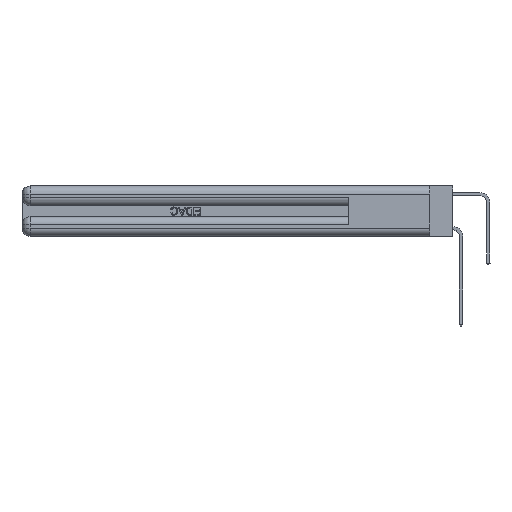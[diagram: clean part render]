
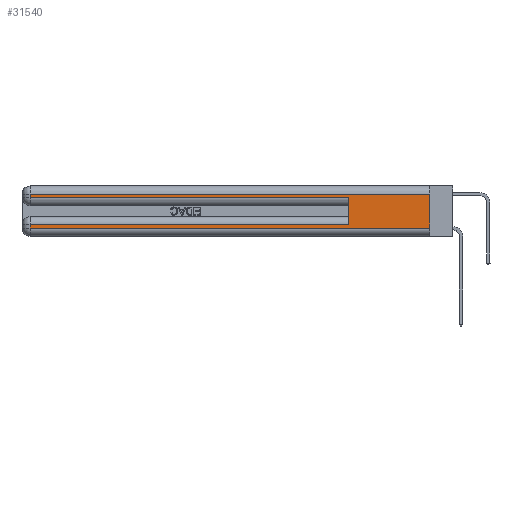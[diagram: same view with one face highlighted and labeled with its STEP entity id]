
A CAD part, left-side view. The second image highlights one B-rep face of the part: STEP entity #31540.
In plain terms, the highlighted planar face has unit normal (-1, 0, 0).
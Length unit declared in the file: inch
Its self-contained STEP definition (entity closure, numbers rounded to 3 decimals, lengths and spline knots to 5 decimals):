
#70 = CARTESIAN_POINT ( 'NONE',  ( 0., 0.6, 0.285 ) ) ;
#547 = DIRECTION ( 'NONE',  ( 0., 0., -1. ) ) ;
#630 = CARTESIAN_POINT ( 'NONE',  ( 0., 2.94, 0.06 ) ) ;
#1908 = VERTEX_POINT ( 'NONE', #31203 ) ;
#2025 = AXIS2_PLACEMENT_3D ( 'NONE', #29308, #29480, #26741 ) ;
#2280 = LINE ( 'NONE', #9863, #27321 ) ;
#4072 = ORIENTED_EDGE ( 'NONE', *, *, #21065, .T. ) ;
#4826 = LINE ( 'NONE', #23389, #30517 ) ;
#4921 = LINE ( 'NONE', #17316, #7144 ) ;
#6355 = EDGE_CURVE ( 'NONE', #16279, #23256, #4921, .T. ) ;
#6655 = EDGE_CURVE ( 'NONE', #13096, #23256, #31890, .T. ) ;
#7144 = VECTOR ( 'NONE', #25375, 39.37008 ) ;
#7744 = VECTOR ( 'NONE', #29300, 39.37008 ) ;
#7885 = CARTESIAN_POINT ( 'NONE',  ( 0., 0., 0.06 ) ) ;
#9117 = VECTOR ( 'NONE', #29813, 39.37008 ) ;
#9369 = ORIENTED_EDGE ( 'NONE', *, *, #16416, .T. ) ;
#9800 = VERTEX_POINT ( 'NONE', #70 ) ;
#9863 = CARTESIAN_POINT ( 'NONE',  ( 0., 0., 0.085 ) ) ;
#10350 = LINE ( 'NONE', #33690, #14319 ) ;
#11595 = CARTESIAN_POINT ( 'NONE',  ( 0., 2.94, 0.31 ) ) ;
#12131 = ORIENTED_EDGE ( 'NONE', *, *, #6355, .T. ) ;
#12452 = DIRECTION ( 'NONE',  ( 0., 1., 0. ) ) ;
#13096 = VERTEX_POINT ( 'NONE', #29073 ) ;
#14130 = VERTEX_POINT ( 'NONE', #26867 ) ;
#14319 = VECTOR ( 'NONE', #31304, 39.37008 ) ;
#14481 = EDGE_CURVE ( 'NONE', #18541, #16279, #24759, .T. ) ;
#16017 = VECTOR ( 'NONE', #33556, 39.37008 ) ;
#16279 = VERTEX_POINT ( 'NONE', #630 ) ;
#16416 = EDGE_CURVE ( 'NONE', #1908, #18541, #2280, .T. ) ;
#17316 = CARTESIAN_POINT ( 'NONE',  ( 0., 0., 0.06 ) ) ;
#17432 = ORIENTED_EDGE ( 'NONE', *, *, #32153, .F. ) ;
#17605 = CARTESIAN_POINT ( 'NONE',  ( 0., 0., 0.285 ) ) ;
#18541 = VERTEX_POINT ( 'NONE', #20766 ) ;
#18839 = CARTESIAN_POINT ( 'NONE',  ( 0., 0., 0.37 ) ) ;
#18846 = PLANE ( 'NONE',  #2025 ) ;
#19350 = CARTESIAN_POINT ( 'NONE',  ( 0., 0.6, 0.145 ) ) ;
#20766 = CARTESIAN_POINT ( 'NONE',  ( 0., 2.94, 0.085 ) ) ;
#21065 = EDGE_CURVE ( 'NONE', #14130, #9800, #26171, .T. ) ;
#21498 = EDGE_CURVE ( 'NONE', #13096, #30495, #4826, .T. ) ;
#22416 = EDGE_LOOP ( 'NONE', ( #31210, #25229, #33582, #4072, #17432, #9369, #30780, #12131 ) ) ;
#22792 = EDGE_CURVE ( 'NONE', #30495, #14130, #10350, .T. ) ;
#23256 = VERTEX_POINT ( 'NONE', #7885 ) ;
#23389 = CARTESIAN_POINT ( 'NONE',  ( 0., 0., 0.31 ) ) ;
#24759 = LINE ( 'NONE', #27152, #29866 ) ;
#25229 = ORIENTED_EDGE ( 'NONE', *, *, #21498, .T. ) ;
#25375 = DIRECTION ( 'NONE',  ( 0., -1., 0. ) ) ;
#26171 = LINE ( 'NONE', #17605, #16017 ) ;
#26741 = DIRECTION ( 'NONE',  ( 0., 0., -1. ) ) ;
#26867 = CARTESIAN_POINT ( 'NONE',  ( 0., 2.94, 0.285 ) ) ;
#27152 = CARTESIAN_POINT ( 'NONE',  ( 0., 2.94, 0.37 ) ) ;
#27235 = FACE_OUTER_BOUND ( 'NONE', #22416, .T. ) ;
#27321 = VECTOR ( 'NONE', #12452, 39.37008 ) ;
#29073 = CARTESIAN_POINT ( 'NONE',  ( 0., 0., 0.31 ) ) ;
#29300 = DIRECTION ( 'NONE',  ( 0., 0., -1. ) ) ;
#29308 = CARTESIAN_POINT ( 'NONE',  ( 0., 0., 0.37 ) ) ;
#29480 = DIRECTION ( 'NONE',  ( 1., 0., 0. ) ) ;
#29813 = DIRECTION ( 'NONE',  ( 0., 0., 1. ) ) ;
#29866 = VECTOR ( 'NONE', #547, 39.37008 ) ;
#30495 = VERTEX_POINT ( 'NONE', #11595 ) ;
#30517 = VECTOR ( 'NONE', #33866, 39.37008 ) ;
#30780 = ORIENTED_EDGE ( 'NONE', *, *, #14481, .T. ) ;
#31203 = CARTESIAN_POINT ( 'NONE',  ( 0., 0.6, 0.085 ) ) ;
#31210 = ORIENTED_EDGE ( 'NONE', *, *, #6655, .F. ) ;
#31304 = DIRECTION ( 'NONE',  ( 0., 0., -1. ) ) ;
#31540 = ADVANCED_FACE ( 'NONE', ( #27235 ), #18846, .F. ) ;
#31890 = LINE ( 'NONE', #18839, #7744 ) ;
#32153 = EDGE_CURVE ( 'NONE', #1908, #9800, #32405, .T. ) ;
#32405 = LINE ( 'NONE', #19350, #9117 ) ;
#33556 = DIRECTION ( 'NONE',  ( 0., -1., 0. ) ) ;
#33582 = ORIENTED_EDGE ( 'NONE', *, *, #22792, .T. ) ;
#33690 = CARTESIAN_POINT ( 'NONE',  ( 0., 2.94, 0.37 ) ) ;
#33866 = DIRECTION ( 'NONE',  ( 0., 1., 0. ) ) ;
